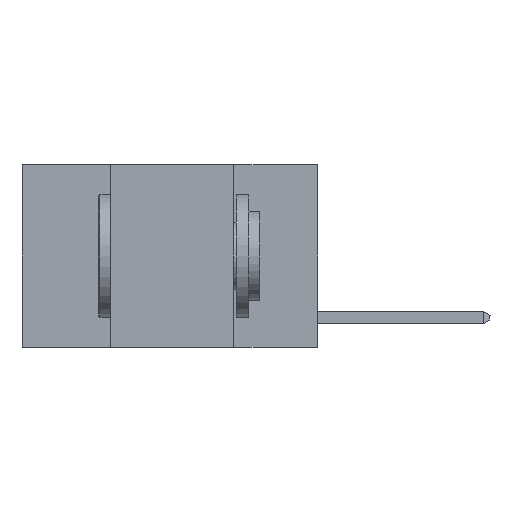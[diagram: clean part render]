
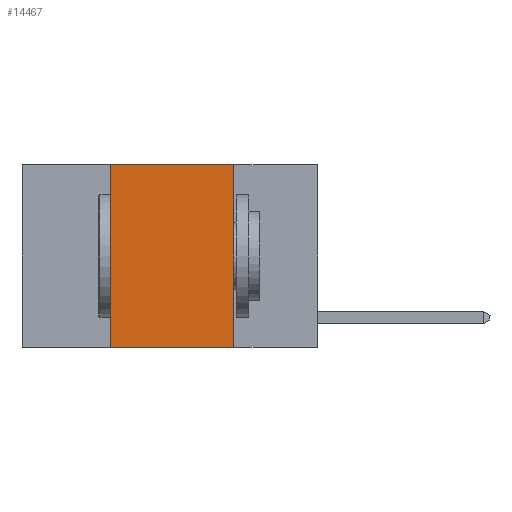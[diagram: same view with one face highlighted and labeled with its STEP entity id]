
A CAD part, left-side view. The second image highlights one B-rep face of the part: STEP entity #14467.
In plain terms, the highlighted planar face has unit normal (-1, 0, 0).
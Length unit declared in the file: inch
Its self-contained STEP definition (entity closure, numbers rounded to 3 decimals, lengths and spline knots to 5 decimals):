
#119 = LINE ( 'NONE', #11723, #13755 ) ;
#466 = ORIENTED_EDGE ( 'NONE', *, *, #15839, .F. ) ;
#905 = EDGE_CURVE ( 'NONE', #20323, #12537, #23306, .T. ) ;
#2300 = AXIS2_PLACEMENT_3D ( 'NONE', #19598, #13602, #3782 ) ;
#2460 = CARTESIAN_POINT ( 'NONE',  ( 0., 0.42, -0.37 ) ) ;
#2713 = CARTESIAN_POINT ( 'NONE',  ( 0., 0.42, 0. ) ) ;
#2847 = EDGE_LOOP ( 'NONE', ( #466, #8272, #17080, #12494 ) ) ;
#3782 = DIRECTION ( 'NONE',  ( 0., 0., -1. ) ) ;
#4352 = EDGE_CURVE ( 'NONE', #20323, #19751, #119, .T. ) ;
#6306 = CARTESIAN_POINT ( 'NONE',  ( 0., 0.17, 0. ) ) ;
#6697 = VECTOR ( 'NONE', #8745, 39.37008 ) ;
#7339 = LINE ( 'NONE', #6306, #15385 ) ;
#8272 = ORIENTED_EDGE ( 'NONE', *, *, #25509, .F. ) ;
#8745 = DIRECTION ( 'NONE',  ( 0., 0., 1. ) ) ;
#10169 = DIRECTION ( 'NONE',  ( 0., -1., 0. ) ) ;
#11606 = CARTESIAN_POINT ( 'NONE',  ( 0., 0.17, -0.37 ) ) ;
#11723 = CARTESIAN_POINT ( 'NONE',  ( 0., 0.6, -0.37 ) ) ;
#12061 = DIRECTION ( 'NONE',  ( 0., 0., -1. ) ) ;
#12218 = CARTESIAN_POINT ( 'NONE',  ( 0., 0.6, 0. ) ) ;
#12494 = ORIENTED_EDGE ( 'NONE', *, *, #4352, .T. ) ;
#12537 = VERTEX_POINT ( 'NONE', #19300 ) ;
#12626 = CARTESIAN_POINT ( 'NONE',  ( 0., 0.17, 0. ) ) ;
#13602 = DIRECTION ( 'NONE',  ( 1., 0., 0. ) ) ;
#13755 = VECTOR ( 'NONE', #10169, 39.37008 ) ;
#13821 = VERTEX_POINT ( 'NONE', #12626 ) ;
#14467 = ADVANCED_FACE ( 'NONE', ( #18907 ), #15527, .F. ) ;
#15385 = VECTOR ( 'NONE', #12061, 39.37008 ) ;
#15527 = PLANE ( 'NONE',  #2300 ) ;
#15839 = EDGE_CURVE ( 'NONE', #13821, #19751, #7339, .T. ) ;
#17080 = ORIENTED_EDGE ( 'NONE', *, *, #905, .F. ) ;
#18572 = DIRECTION ( 'NONE',  ( 0., -1., 0. ) ) ;
#18907 = FACE_OUTER_BOUND ( 'NONE', #2847, .T. ) ;
#19300 = CARTESIAN_POINT ( 'NONE',  ( 0., 0.42, 0. ) ) ;
#19598 = CARTESIAN_POINT ( 'NONE',  ( 0., 0.6, 0. ) ) ;
#19751 = VERTEX_POINT ( 'NONE', #11606 ) ;
#20323 = VERTEX_POINT ( 'NONE', #2460 ) ;
#21205 = LINE ( 'NONE', #12218, #22491 ) ;
#22491 = VECTOR ( 'NONE', #18572, 39.37008 ) ;
#23306 = LINE ( 'NONE', #2713, #6697 ) ;
#25509 = EDGE_CURVE ( 'NONE', #12537, #13821, #21205, .T. ) ;
